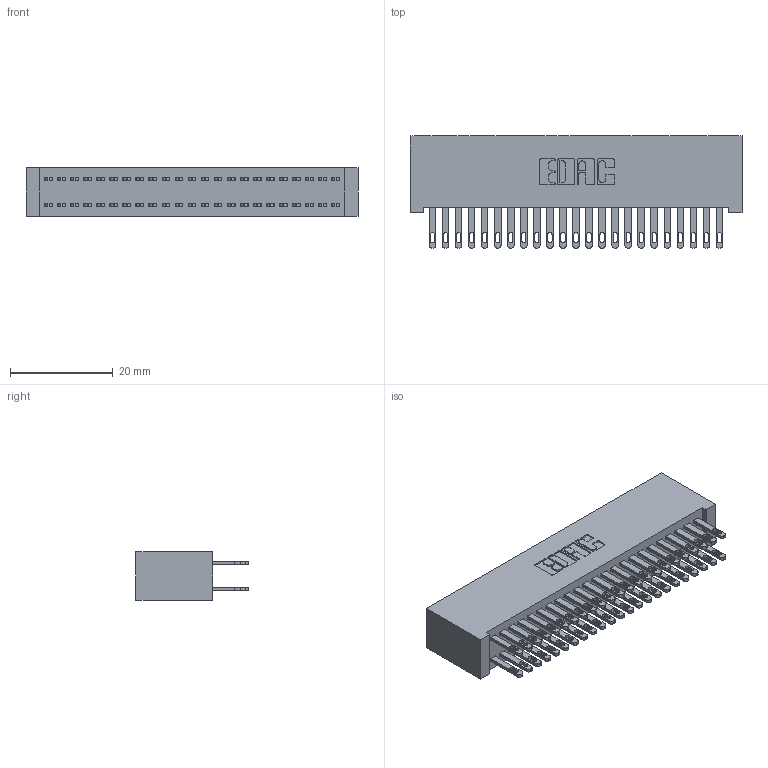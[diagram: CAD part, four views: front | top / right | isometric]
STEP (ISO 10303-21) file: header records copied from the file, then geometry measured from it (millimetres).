
FILE_DESCRIPTION (( 'STEP AP203' ), '1' );
FILE_NAME ('892-046-500-201.STEP', '2020-09-21T17:16:06', ( '' ), ( '' ), 'SwSTEP 2.0', 'SolidWorks 2020', '' );
FILE_SCHEMA (( 'CONFIG_CONTROL_DESIGN' ));
Length unit declared in the file: inch
Products named in the file (3): 345-292-001_345-293-100; 842 Part_Lugless; 892-046-500-201
Assembly tree (47 placements, depth 2):
  892-046-500-201
    842 Part_Lugless
    345-292-001_345-293-100  x46
Bounding box: 64.67 x 21.85 x 9.4 mm (x, y, z)
Volume: 6300.6 mm3; surface area: 10674.3 mm2
Topology: 47 solids, 47 shells, 2310 faces, 7037 edges, 4690 vertices
Faces by surface type: plane 1442, cylinder 868
Entity records: 16775 total; most frequent: CARTESIAN_POINT 2798, ORIENTED_EDGE 2734, DIRECTION 2419, EDGE_CURVE 1367, VECTOR 1243, LINE 1243, VERTEX_POINT 910, AXIS2_PLACEMENT_3D 588
